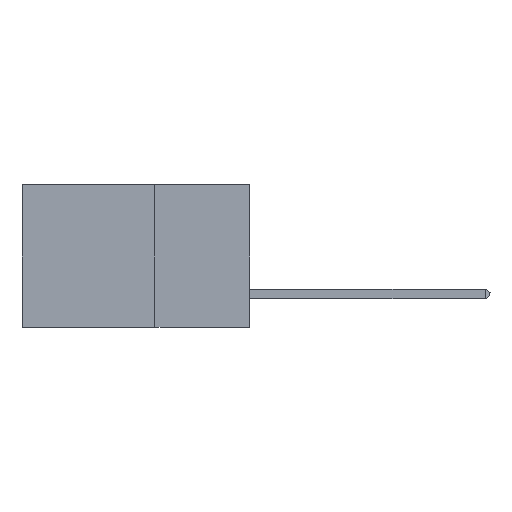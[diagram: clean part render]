
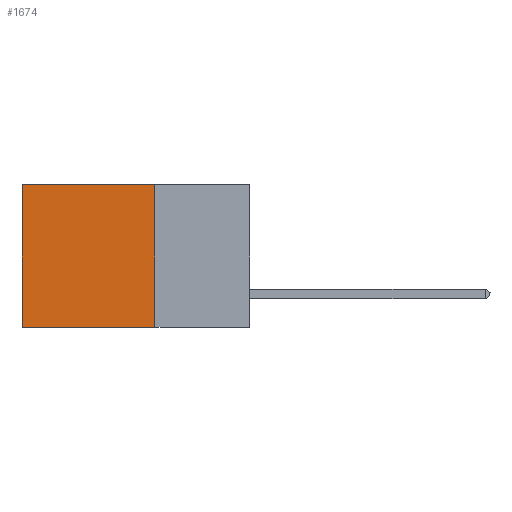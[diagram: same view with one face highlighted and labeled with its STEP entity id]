
A CAD part, left-side view. The second image highlights one B-rep face of the part: STEP entity #1674.
In plain terms, the highlighted planar face has unit normal (-1, 0, 0).
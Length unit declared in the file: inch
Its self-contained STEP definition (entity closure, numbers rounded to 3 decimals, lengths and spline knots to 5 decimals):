
#387 = PLANE ( 'NONE',  #12228 ) ;
#444 = LINE ( 'NONE', #2484, #9158 ) ;
#1067 = VECTOR ( 'NONE', #6295, 39.37008 ) ;
#1247 = ORIENTED_EDGE ( 'NONE', *, *, #3282, .T. ) ;
#1674 = ADVANCED_FACE ( 'NONE', ( #8304 ), #387, .F. ) ;
#1686 = LINE ( 'NONE', #10565, #13776 ) ;
#1850 = CARTESIAN_POINT ( 'NONE',  ( 0.2875, 0.25, 0. ) ) ;
#1939 = LINE ( 'NONE', #11838, #1067 ) ;
#2484 = CARTESIAN_POINT ( 'NONE',  ( 0.2875, 0.25, -0.375 ) ) ;
#2498 = CARTESIAN_POINT ( 'NONE',  ( 0.2875, 0.25, -0.375 ) ) ;
#2726 = VERTEX_POINT ( 'NONE', #13485 ) ;
#2866 = DIRECTION ( 'NONE',  ( 0., 1., 0. ) ) ;
#2906 = EDGE_CURVE ( 'NONE', #9051, #4618, #1939, .T. ) ;
#3282 = EDGE_CURVE ( 'NONE', #2726, #6145, #5124, .T. ) ;
#4618 = VERTEX_POINT ( 'NONE', #10801 ) ;
#4830 = DIRECTION ( 'NONE',  ( 1., 0., 0. ) ) ;
#5034 = DIRECTION ( 'NONE',  ( 0., 0., -1. ) ) ;
#5124 = LINE ( 'NONE', #1850, #11754 ) ;
#6145 = VERTEX_POINT ( 'NONE', #8380 ) ;
#6295 = DIRECTION ( 'NONE',  ( 0., 1., 0. ) ) ;
#6688 = EDGE_LOOP ( 'NONE', ( #13263, #11187, #7810, #1247 ) ) ;
#6913 = DIRECTION ( 'NONE',  ( 0., 0., -1. ) ) ;
#6996 = DIRECTION ( 'NONE',  ( 0., 0., -1. ) ) ;
#7810 = ORIENTED_EDGE ( 'NONE', *, *, #12855, .F. ) ;
#8304 = FACE_OUTER_BOUND ( 'NONE', #6688, .T. ) ;
#8380 = CARTESIAN_POINT ( 'NONE',  ( 0.2875, 0.6, 0. ) ) ;
#8387 = CARTESIAN_POINT ( 'NONE',  ( 0.2875, 0.25, -0.375 ) ) ;
#9051 = VERTEX_POINT ( 'NONE', #8387 ) ;
#9158 = VECTOR ( 'NONE', #6913, 39.37008 ) ;
#9478 = EDGE_CURVE ( 'NONE', #6145, #4618, #1686, .T. ) ;
#10565 = CARTESIAN_POINT ( 'NONE',  ( 0.2875, 0.6, -0.375 ) ) ;
#10801 = CARTESIAN_POINT ( 'NONE',  ( 0.2875, 0.6, -0.375 ) ) ;
#11187 = ORIENTED_EDGE ( 'NONE', *, *, #2906, .F. ) ;
#11754 = VECTOR ( 'NONE', #2866, 39.37008 ) ;
#11838 = CARTESIAN_POINT ( 'NONE',  ( 0.2875, 0.25, -0.375 ) ) ;
#12228 = AXIS2_PLACEMENT_3D ( 'NONE', #2498, #4830, #6996 ) ;
#12855 = EDGE_CURVE ( 'NONE', #2726, #9051, #444, .T. ) ;
#13263 = ORIENTED_EDGE ( 'NONE', *, *, #9478, .T. ) ;
#13485 = CARTESIAN_POINT ( 'NONE',  ( 0.2875, 0.25, 0. ) ) ;
#13776 = VECTOR ( 'NONE', #5034, 39.37008 ) ;
